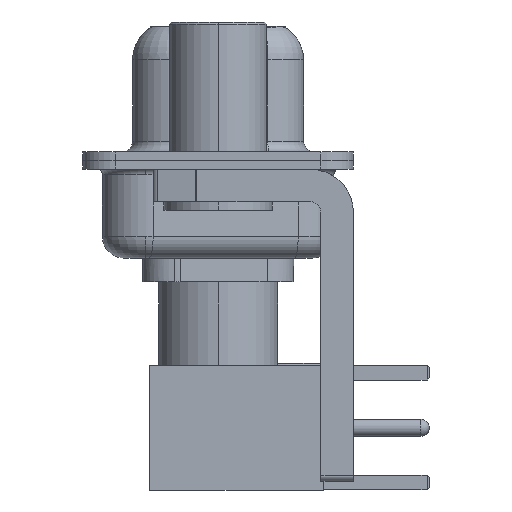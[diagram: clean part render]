
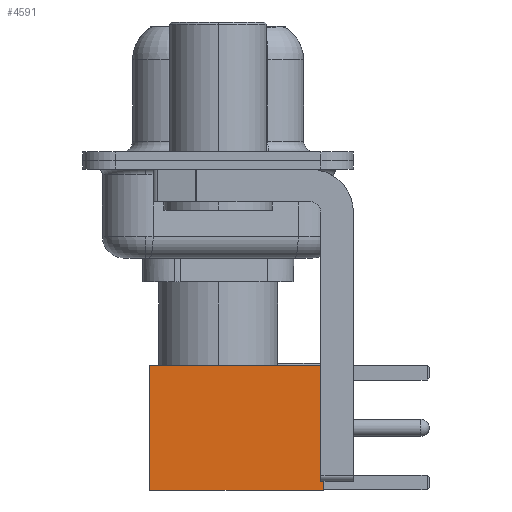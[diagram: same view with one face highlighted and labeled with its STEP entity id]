
A CAD part, left-side view. The second image highlights one B-rep face of the part: STEP entity #4591.
In plain terms, the highlighted face is planar.
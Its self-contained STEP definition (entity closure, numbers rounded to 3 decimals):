
#61 = AXIS2_PLACEMENT_3D ( 'NONE', #10353, #8591, #10487 ) ;
#1274 = DIRECTION ( 'NONE',  ( -1., 0., 0. ) ) ;
#1432 = EDGE_CURVE ( 'NONE', #11790, #2952, #7232, .T. ) ;
#2952 = VERTEX_POINT ( 'NONE', #25409 ) ;
#4591 = ADVANCED_FACE ( 'NONE', ( #21181 ), #14404, .T. ) ;
#4706 = CARTESIAN_POINT ( 'NONE',  ( 2.875, 2.875, 8. ) ) ;
#5541 = VERTEX_POINT ( 'NONE', #4706 ) ;
#6239 = LINE ( 'NONE', #18283, #14733 ) ;
#7232 = LINE ( 'NONE', #13430, #16666 ) ;
#8493 = LINE ( 'NONE', #12946, #14825 ) ;
#8591 = DIRECTION ( 'NONE',  ( 0., 1., 0. ) ) ;
#8819 = ORIENTED_EDGE ( 'NONE', *, *, #1432, .T. ) ;
#10353 = CARTESIAN_POINT ( 'NONE',  ( 2.875, 2.875, 0. ) ) ;
#10435 = ORIENTED_EDGE ( 'NONE', *, *, #22020, .T. ) ;
#10487 = DIRECTION ( 'NONE',  ( 0., 0., 1. ) ) ;
#11058 = ORIENTED_EDGE ( 'NONE', *, *, #13988, .F. ) ;
#11790 = VERTEX_POINT ( 'NONE', #20666 ) ;
#11889 = EDGE_CURVE ( 'NONE', #17292, #2952, #8493, .T. ) ;
#12946 = CARTESIAN_POINT ( 'NONE',  ( -2.875, 2.875, 0. ) ) ;
#13430 = CARTESIAN_POINT ( 'NONE',  ( 0., 2.875, 0. ) ) ;
#13988 = EDGE_CURVE ( 'NONE', #5541, #17292, #17659, .T. ) ;
#14404 = PLANE ( 'NONE',  #61 ) ;
#14733 = VECTOR ( 'NONE', #20056, 1000. ) ;
#14825 = VECTOR ( 'NONE', #21087, 1000. ) ;
#16333 = CARTESIAN_POINT ( 'NONE',  ( -2.875, 2.875, 8. ) ) ;
#16666 = VECTOR ( 'NONE', #1274, 1000. ) ;
#17292 = VERTEX_POINT ( 'NONE', #16333 ) ;
#17659 = LINE ( 'NONE', #23909, #18363 ) ;
#18283 = CARTESIAN_POINT ( 'NONE',  ( 2.875, 2.875, 0. ) ) ;
#18363 = VECTOR ( 'NONE', #23643, 1000. ) ;
#20056 = DIRECTION ( 'NONE',  ( 0., 0., -1. ) ) ;
#20666 = CARTESIAN_POINT ( 'NONE',  ( 2.875, 2.875, 0. ) ) ;
#20860 = EDGE_LOOP ( 'NONE', ( #10435, #8819, #22132, #11058 ) ) ;
#21087 = DIRECTION ( 'NONE',  ( 0., 0., -1. ) ) ;
#21181 = FACE_OUTER_BOUND ( 'NONE', #20860, .T. ) ;
#22020 = EDGE_CURVE ( 'NONE', #5541, #11790, #6239, .T. ) ;
#22132 = ORIENTED_EDGE ( 'NONE', *, *, #11889, .F. ) ;
#23643 = DIRECTION ( 'NONE',  ( -1., 0., 0. ) ) ;
#23909 = CARTESIAN_POINT ( 'NONE',  ( 0., 2.875, 8. ) ) ;
#25409 = CARTESIAN_POINT ( 'NONE',  ( -2.875, 2.875, 0. ) ) ;
